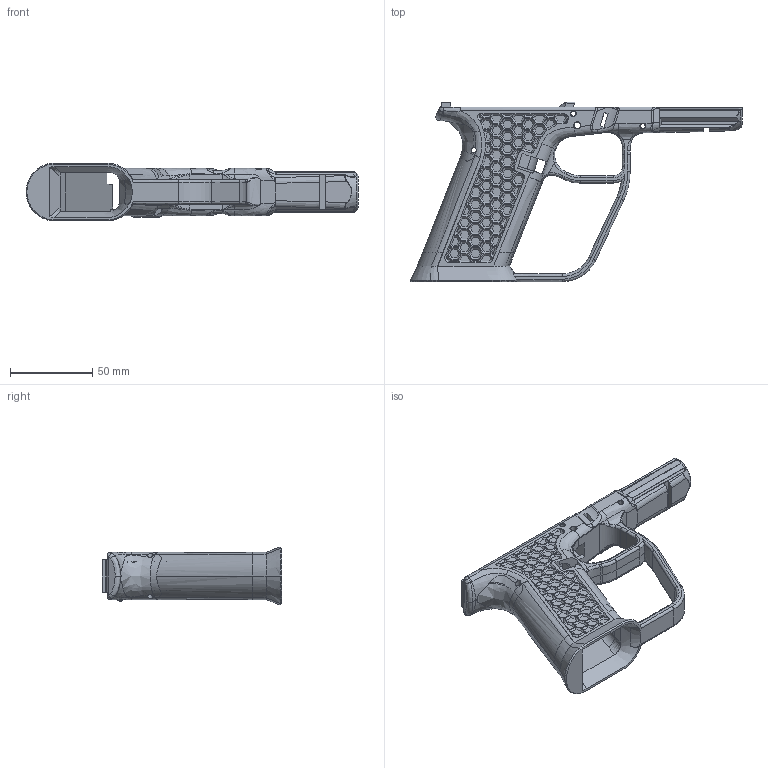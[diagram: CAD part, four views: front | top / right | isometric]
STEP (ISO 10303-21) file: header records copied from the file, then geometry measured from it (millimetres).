
FILE_DESCRIPTION(/* description */ (''),/* implementation_level */ '2;1');
FILE_NAME(/* name */ 'SG17.2.step',/* time_stamp */ '2021-01-21T02:26:56-06:00',/* author */ (''),/* organization */ (''),/* preprocessor_version */ 'ST-DEVELOPER v18.1',/* originating_system */ 'Autodesk Translation Framework v9.7.1.1290',/* authorisation */ '');
FILE_SCHEMA (('AUTOMOTIVE_DESIGN { 1 0 10303 214 3 1 1 }'));
Products named in the file (1): FMDA DD17.2 v1.4 SFG
Bounding box: 202.12 x 109.21 x 35.29 mm (x, y, z)
Volume: 92941.2 mm3; surface area: 53392.1 mm2
Topology: 2 solids, 4 shells, 1677 faces, 4403 edges, 2865 vertices
Faces by surface type: plane 1167, bspline 296, cylinder 123, cone 58, torus 17, sphere 16
Full cylindrical faces by diameter (mm): 2 x1, 3 x4, 3.2 x2, 4 x2
Entity records: 77169 total; most frequent: CARTESIAN_POINT 37718, ORIENTED_EDGE 8788, DIRECTION 7039, EDGE_CURVE 4394, LINE 3187, VECTOR 3187, VERTEX_POINT 2865, AXIS2_PLACEMENT_3D 1926
